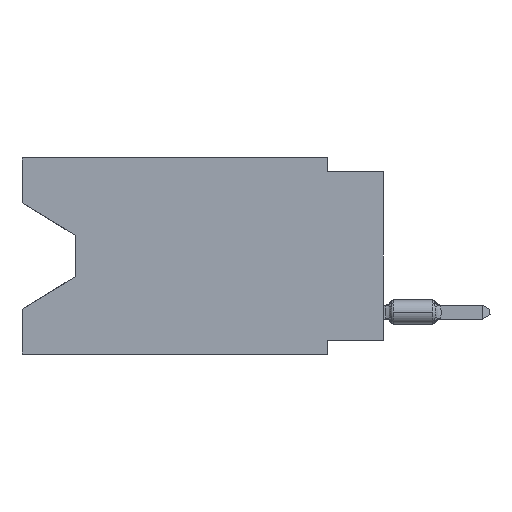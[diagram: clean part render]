
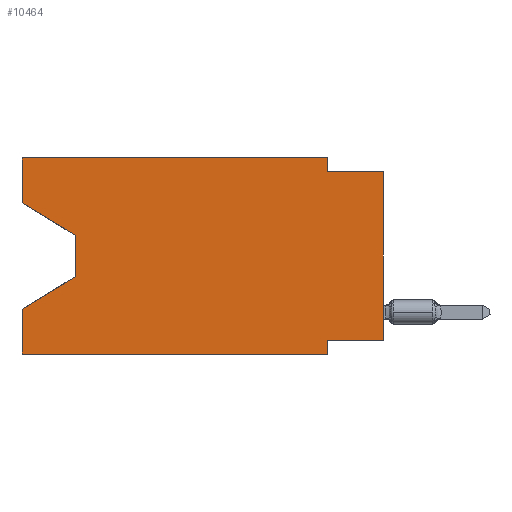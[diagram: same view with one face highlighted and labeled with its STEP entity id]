
A CAD part, left-side view. The second image highlights one B-rep face of the part: STEP entity #10464.
In plain terms, the highlighted planar face has unit normal (-1, 0, 0).
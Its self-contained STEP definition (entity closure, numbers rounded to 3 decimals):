
#145 = EDGE_LOOP ( 'NONE', ( #21840, #35176, #44424, #28434, #37896, #7105, #23455, #50119, #16359, #43639, #5133, #32853 ) ) ;
#829 = CARTESIAN_POINT ( 'NONE',  ( 0., 16.383, -8.89 ) ) ;
#1639 = CARTESIAN_POINT ( 'NONE',  ( 0., 2.54, -8.255 ) ) ;
#1932 = EDGE_CURVE ( 'NONE', #17806, #22963, #32171, .T. ) ;
#2204 = PLANE ( 'NONE',  #33045 ) ;
#3776 = CARTESIAN_POINT ( 'NONE',  ( 0., 0., -0.635 ) ) ;
#4027 = EDGE_CURVE ( 'NONE', #6204, #16957, #12983, .T. ) ;
#4785 = VECTOR ( 'NONE', #8998, 1000. ) ;
#5133 = ORIENTED_EDGE ( 'NONE', *, *, #48360, .F. ) ;
#5535 = VERTEX_POINT ( 'NONE', #8954 ) ;
#5636 = DIRECTION ( 'NONE',  ( 0., 0., -1. ) ) ;
#5888 = CARTESIAN_POINT ( 'NONE',  ( 0., 13.97, -5.385 ) ) ;
#6132 = CARTESIAN_POINT ( 'NONE',  ( 0., 2.54, -8.89 ) ) ;
#6204 = VERTEX_POINT ( 'NONE', #13810 ) ;
#6314 = FACE_OUTER_BOUND ( 'NONE', #145, .T. ) ;
#7105 = ORIENTED_EDGE ( 'NONE', *, *, #17852, .F. ) ;
#8954 = CARTESIAN_POINT ( 'NONE',  ( 0., 16.383, -2.038 ) ) ;
#8998 = DIRECTION ( 'NONE',  ( 0., 0., -1. ) ) ;
#9470 = EDGE_CURVE ( 'NONE', #48373, #48989, #15591, .T. ) ;
#10031 = LINE ( 'NONE', #6132, #12908 ) ;
#10212 = CARTESIAN_POINT ( 'NONE',  ( 0., 16.383, 0. ) ) ;
#10464 = ADVANCED_FACE ( 'NONE', ( #6314 ), #2204, .F. ) ;
#12908 = VECTOR ( 'NONE', #5636, 1000. ) ;
#12909 = LINE ( 'NONE', #28675, #4785 ) ;
#12983 = LINE ( 'NONE', #40425, #25894 ) ;
#13810 = CARTESIAN_POINT ( 'NONE',  ( 0., 0., -8.255 ) ) ;
#15332 = CARTESIAN_POINT ( 'NONE',  ( 0., 16.383, 0. ) ) ;
#15591 = LINE ( 'NONE', #46923, #18142 ) ;
#16292 = VECTOR ( 'NONE', #45638, 1000. ) ;
#16359 = ORIENTED_EDGE ( 'NONE', *, *, #9470, .F. ) ;
#16479 = DIRECTION ( 'NONE',  ( 0., -0.855, -0.519 ) ) ;
#16957 = VERTEX_POINT ( 'NONE', #1639 ) ;
#17806 = VERTEX_POINT ( 'NONE', #5888 ) ;
#17852 = EDGE_CURVE ( 'NONE', #16957, #24792, #10031, .T. ) ;
#18142 = VECTOR ( 'NONE', #50290, 1000. ) ;
#19165 = CARTESIAN_POINT ( 'NONE',  ( 0., 2.54, 0. ) ) ;
#19792 = EDGE_CURVE ( 'NONE', #36657, #48373, #12909, .T. ) ;
#21515 = EDGE_CURVE ( 'NONE', #5535, #25844, #24752, .T. ) ;
#21840 = ORIENTED_EDGE ( 'NONE', *, *, #21515, .T. ) ;
#21925 = VECTOR ( 'NONE', #36057, 1000. ) ;
#22149 = DIRECTION ( 'NONE',  ( 0., 0., -1. ) ) ;
#22556 = DIRECTION ( 'NONE',  ( 0., 0., 1. ) ) ;
#22963 = VERTEX_POINT ( 'NONE', #42754 ) ;
#23455 = ORIENTED_EDGE ( 'NONE', *, *, #4027, .F. ) ;
#24196 = EDGE_CURVE ( 'NONE', #25844, #17806, #44348, .T. ) ;
#24674 = CARTESIAN_POINT ( 'NONE',  ( 0., 13.97, -3.505 ) ) ;
#24752 = LINE ( 'NONE', #40543, #25475 ) ;
#24792 = VERTEX_POINT ( 'NONE', #26880 ) ;
#25304 = VECTOR ( 'NONE', #48060, 1000. ) ;
#25475 = VECTOR ( 'NONE', #16479, 1000. ) ;
#25476 = VECTOR ( 'NONE', #40965, 1000. ) ;
#25844 = VERTEX_POINT ( 'NONE', #37653 ) ;
#25894 = VECTOR ( 'NONE', #29263, 1000. ) ;
#26880 = CARTESIAN_POINT ( 'NONE',  ( 0., 2.54, -8.89 ) ) ;
#27048 = EDGE_CURVE ( 'NONE', #6204, #48989, #35310, .T. ) ;
#28012 = CARTESIAN_POINT ( 'NONE',  ( 0., 13.97, -5.385 ) ) ;
#28434 = ORIENTED_EDGE ( 'NONE', *, *, #42646, .F. ) ;
#28675 = CARTESIAN_POINT ( 'NONE',  ( 0., 2.54, 0. ) ) ;
#29065 = VECTOR ( 'NONE', #40447, 1000. ) ;
#29263 = DIRECTION ( 'NONE',  ( 0., 1., 0. ) ) ;
#29570 = CARTESIAN_POINT ( 'NONE',  ( 0., 2.54, -0.635 ) ) ;
#30187 = EDGE_CURVE ( 'NONE', #5535, #50868, #38088, .T. ) ;
#31014 = VERTEX_POINT ( 'NONE', #46447 ) ;
#31745 = LINE ( 'NONE', #35126, #25304 ) ;
#32171 = LINE ( 'NONE', #28012, #29065 ) ;
#32853 = ORIENTED_EDGE ( 'NONE', *, *, #30187, .F. ) ;
#33045 = AXIS2_PLACEMENT_3D ( 'NONE', #10212, #49338, #22149 ) ;
#33828 = EDGE_CURVE ( 'NONE', #31014, #24792, #40452, .T. ) ;
#34467 = CARTESIAN_POINT ( 'NONE',  ( 0., 16.383, 0. ) ) ;
#35126 = CARTESIAN_POINT ( 'NONE',  ( 0., 16.383, 0. ) ) ;
#35176 = ORIENTED_EDGE ( 'NONE', *, *, #24196, .T. ) ;
#35310 = LINE ( 'NONE', #39193, #48715 ) ;
#36057 = DIRECTION ( 'NONE',  ( 0., -1., 0. ) ) ;
#36657 = VERTEX_POINT ( 'NONE', #19165 ) ;
#37653 = CARTESIAN_POINT ( 'NONE',  ( 0., 13.97, -3.505 ) ) ;
#37896 = ORIENTED_EDGE ( 'NONE', *, *, #33828, .T. ) ;
#38088 = LINE ( 'NONE', #34467, #49054 ) ;
#39193 = CARTESIAN_POINT ( 'NONE',  ( 0., 0., 0. ) ) ;
#40425 = CARTESIAN_POINT ( 'NONE',  ( 0., 0., -8.255 ) ) ;
#40447 = DIRECTION ( 'NONE',  ( 0., 0.855, -0.519 ) ) ;
#40452 = LINE ( 'NONE', #829, #21925 ) ;
#40543 = CARTESIAN_POINT ( 'NONE',  ( 0., 16.383, -2.038 ) ) ;
#40965 = DIRECTION ( 'NONE',  ( 0., 0., -1. ) ) ;
#42497 = LINE ( 'NONE', #46140, #16292 ) ;
#42564 = DIRECTION ( 'NONE',  ( 0., 0., 1. ) ) ;
#42646 = EDGE_CURVE ( 'NONE', #31014, #22963, #31745, .T. ) ;
#42754 = CARTESIAN_POINT ( 'NONE',  ( 0., 16.383, -6.852 ) ) ;
#43639 = ORIENTED_EDGE ( 'NONE', *, *, #19792, .F. ) ;
#44348 = LINE ( 'NONE', #24674, #25476 ) ;
#44424 = ORIENTED_EDGE ( 'NONE', *, *, #1932, .T. ) ;
#45638 = DIRECTION ( 'NONE',  ( 0., -1., 0. ) ) ;
#46140 = CARTESIAN_POINT ( 'NONE',  ( 0., 16.383, 0. ) ) ;
#46447 = CARTESIAN_POINT ( 'NONE',  ( 0., 16.383, -8.89 ) ) ;
#46923 = CARTESIAN_POINT ( 'NONE',  ( 0., 0., -0.635 ) ) ;
#48060 = DIRECTION ( 'NONE',  ( 0., 0., 1. ) ) ;
#48360 = EDGE_CURVE ( 'NONE', #50868, #36657, #42497, .T. ) ;
#48373 = VERTEX_POINT ( 'NONE', #29570 ) ;
#48715 = VECTOR ( 'NONE', #42564, 1000. ) ;
#48989 = VERTEX_POINT ( 'NONE', #3776 ) ;
#49054 = VECTOR ( 'NONE', #22556, 1000. ) ;
#49338 = DIRECTION ( 'NONE',  ( 1., 0., 0. ) ) ;
#50119 = ORIENTED_EDGE ( 'NONE', *, *, #27048, .T. ) ;
#50290 = DIRECTION ( 'NONE',  ( 0., -1., 0. ) ) ;
#50868 = VERTEX_POINT ( 'NONE', #15332 ) ;
